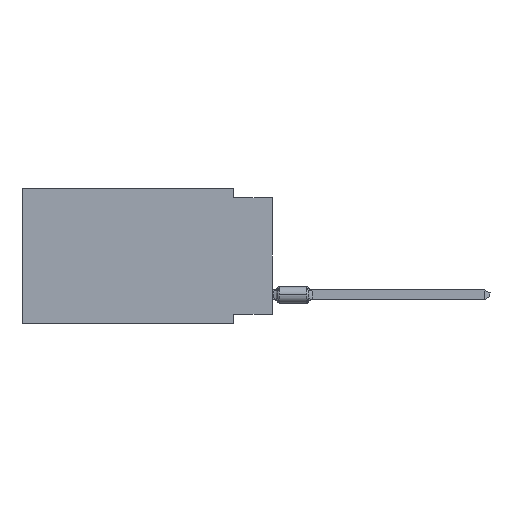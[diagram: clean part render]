
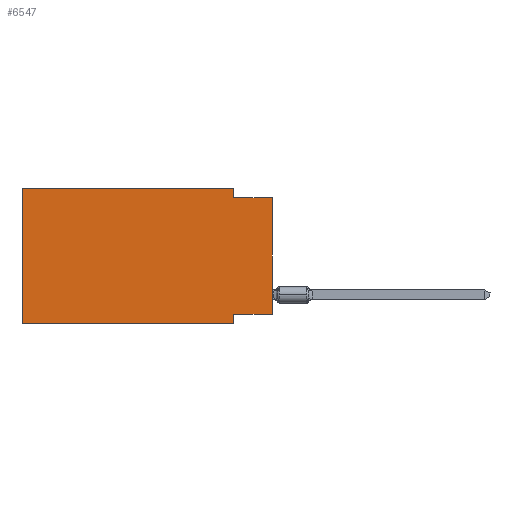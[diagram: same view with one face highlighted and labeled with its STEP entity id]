
A CAD part, left-side view. The second image highlights one B-rep face of the part: STEP entity #6547.
In plain terms, the highlighted planar face has unit normal (-1, 0, 0).
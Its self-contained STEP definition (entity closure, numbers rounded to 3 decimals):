
#294 = VECTOR ( 'NONE', #20735, 1000. ) ;
#1752 = EDGE_CURVE ( 'NONE', #27755, #18205, #9576, .T. ) ;
#1855 = DIRECTION ( 'NONE',  ( 0., 0., -1. ) ) ;
#2251 = VECTOR ( 'NONE', #4967, 1000. ) ;
#2712 = ORIENTED_EDGE ( 'NONE', *, *, #1752, .F. ) ;
#3345 = CARTESIAN_POINT ( 'NONE',  ( 0., 2.54, -8.89 ) ) ;
#4549 = LINE ( 'NONE', #26313, #2251 ) ;
#4967 = DIRECTION ( 'NONE',  ( 0., 0., 1. ) ) ;
#5986 = CARTESIAN_POINT ( 'NONE',  ( 0., 16.383, -8.89 ) ) ;
#6278 = CARTESIAN_POINT ( 'NONE',  ( 0., 16.383, 0. ) ) ;
#6547 = ADVANCED_FACE ( 'NONE', ( #15392 ), #18649, .F. ) ;
#7090 = VECTOR ( 'NONE', #25117, 1000. ) ;
#9576 = LINE ( 'NONE', #6278, #23134 ) ;
#10091 = VECTOR ( 'NONE', #33780, 1000. ) ;
#10302 = ORIENTED_EDGE ( 'NONE', *, *, #21419, .F. ) ;
#10453 = VERTEX_POINT ( 'NONE', #33695 ) ;
#11646 = EDGE_CURVE ( 'NONE', #18205, #21411, #32687, .T. ) ;
#12729 = VERTEX_POINT ( 'NONE', #3345 ) ;
#13380 = EDGE_CURVE ( 'NONE', #37502, #10453, #4549, .T. ) ;
#14409 = ORIENTED_EDGE ( 'NONE', *, *, #18504, .F. ) ;
#15392 = FACE_OUTER_BOUND ( 'NONE', #33709, .T. ) ;
#15789 = DIRECTION ( 'NONE',  ( 0., 0., -1. ) ) ;
#16373 = CARTESIAN_POINT ( 'NONE',  ( 0., 2.54, 0. ) ) ;
#17217 = EDGE_CURVE ( 'NONE', #21411, #10453, #27822, .T. ) ;
#17468 = LINE ( 'NONE', #27308, #38600 ) ;
#18205 = VERTEX_POINT ( 'NONE', #16373 ) ;
#18504 = EDGE_CURVE ( 'NONE', #31167, #27755, #31110, .T. ) ;
#18649 = PLANE ( 'NONE',  #20647 ) ;
#18756 = CARTESIAN_POINT ( 'NONE',  ( 0., 0., -8.255 ) ) ;
#18919 = ORIENTED_EDGE ( 'NONE', *, *, #13380, .T. ) ;
#18983 = CARTESIAN_POINT ( 'NONE',  ( 0., 16.383, 0. ) ) ;
#20647 = AXIS2_PLACEMENT_3D ( 'NONE', #21932, #40198, #15789 ) ;
#20735 = DIRECTION ( 'NONE',  ( 0., -1., 0. ) ) ;
#21123 = CARTESIAN_POINT ( 'NONE',  ( 0., 16.383, -8.89 ) ) ;
#21411 = VERTEX_POINT ( 'NONE', #24227 ) ;
#21419 = EDGE_CURVE ( 'NONE', #34114, #12729, #17468, .T. ) ;
#21932 = CARTESIAN_POINT ( 'NONE',  ( 0., 16.383, 0. ) ) ;
#23134 = VECTOR ( 'NONE', #34399, 1000. ) ;
#23214 = EDGE_CURVE ( 'NONE', #31167, #12729, #29778, .T. ) ;
#24227 = CARTESIAN_POINT ( 'NONE',  ( 0., 2.54, -0.635 ) ) ;
#25117 = DIRECTION ( 'NONE',  ( 0., 1., 0. ) ) ;
#25146 = ORIENTED_EDGE ( 'NONE', *, *, #17217, .F. ) ;
#26313 = CARTESIAN_POINT ( 'NONE',  ( 0., 0., 0. ) ) ;
#27308 = CARTESIAN_POINT ( 'NONE',  ( 0., 2.54, -8.89 ) ) ;
#27433 = ORIENTED_EDGE ( 'NONE', *, *, #23214, .T. ) ;
#27630 = DIRECTION ( 'NONE',  ( 0., 0., 1. ) ) ;
#27755 = VERTEX_POINT ( 'NONE', #37722 ) ;
#27822 = LINE ( 'NONE', #28025, #10091 ) ;
#28025 = CARTESIAN_POINT ( 'NONE',  ( 0., 0., -0.635 ) ) ;
#29604 = DIRECTION ( 'NONE',  ( 0., 0., -1. ) ) ;
#29705 = EDGE_CURVE ( 'NONE', #37502, #34114, #40311, .T. ) ;
#29778 = LINE ( 'NONE', #21123, #294 ) ;
#30523 = CARTESIAN_POINT ( 'NONE',  ( 0., 2.54, -8.255 ) ) ;
#31110 = LINE ( 'NONE', #18983, #36814 ) ;
#31167 = VERTEX_POINT ( 'NONE', #5986 ) ;
#31881 = CARTESIAN_POINT ( 'NONE',  ( 0., 2.54, 0. ) ) ;
#32178 = CARTESIAN_POINT ( 'NONE',  ( 0., 0., -8.255 ) ) ;
#32687 = LINE ( 'NONE', #31881, #35738 ) ;
#33695 = CARTESIAN_POINT ( 'NONE',  ( 0., 0., -0.635 ) ) ;
#33709 = EDGE_LOOP ( 'NONE', ( #18919, #25146, #35378, #2712, #14409, #27433, #10302, #36450 ) ) ;
#33780 = DIRECTION ( 'NONE',  ( 0., -1., 0. ) ) ;
#34114 = VERTEX_POINT ( 'NONE', #30523 ) ;
#34399 = DIRECTION ( 'NONE',  ( 0., -1., 0. ) ) ;
#35378 = ORIENTED_EDGE ( 'NONE', *, *, #11646, .F. ) ;
#35738 = VECTOR ( 'NONE', #29604, 1000. ) ;
#36450 = ORIENTED_EDGE ( 'NONE', *, *, #29705, .F. ) ;
#36814 = VECTOR ( 'NONE', #27630, 1000. ) ;
#37502 = VERTEX_POINT ( 'NONE', #32178 ) ;
#37722 = CARTESIAN_POINT ( 'NONE',  ( 0., 16.383, 0. ) ) ;
#38600 = VECTOR ( 'NONE', #1855, 1000. ) ;
#40198 = DIRECTION ( 'NONE',  ( 1., 0., 0. ) ) ;
#40311 = LINE ( 'NONE', #18756, #7090 ) ;
